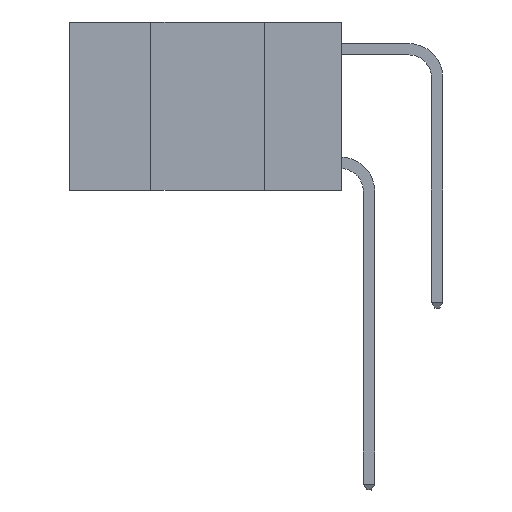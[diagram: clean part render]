
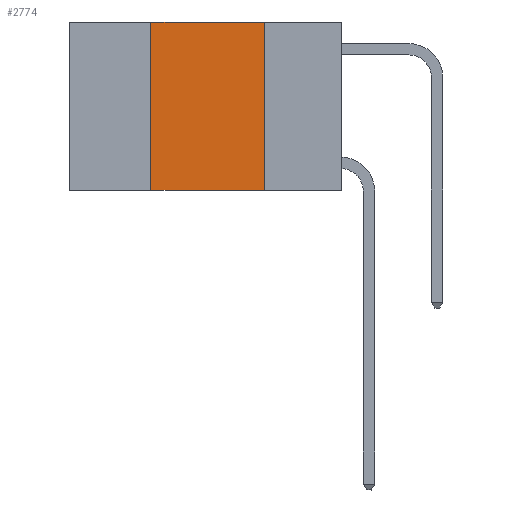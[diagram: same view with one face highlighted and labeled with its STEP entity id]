
A CAD part, left-side view. The second image highlights one B-rep face of the part: STEP entity #2774.
In plain terms, the highlighted planar face has unit normal (-1, 0, 0).
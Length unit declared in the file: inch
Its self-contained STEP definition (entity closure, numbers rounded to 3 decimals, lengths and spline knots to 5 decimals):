
#369 = DIRECTION ( 'NONE',  ( 0., 0., -1. ) ) ;
#434 = CARTESIAN_POINT ( 'NONE',  ( 0., 0.6, 0. ) ) ;
#2393 = LINE ( 'NONE', #25734, #9211 ) ;
#2485 = ORIENTED_EDGE ( 'NONE', *, *, #29262, .F. ) ;
#2774 = ADVANCED_FACE ( 'NONE', ( #15352 ), #8739, .F. ) ;
#2881 = DIRECTION ( 'NONE',  ( 0., 0., 1. ) ) ;
#3376 = CARTESIAN_POINT ( 'NONE',  ( 0., 0.17, 0. ) ) ;
#3693 = DIRECTION ( 'NONE',  ( 1., 0., 0. ) ) ;
#5842 = CARTESIAN_POINT ( 'NONE',  ( 0., 0.6, 0. ) ) ;
#7327 = CARTESIAN_POINT ( 'NONE',  ( 0., 0.42, 0. ) ) ;
#7643 = EDGE_LOOP ( 'NONE', ( #12075, #2485, #14663, #25726 ) ) ;
#8739 = PLANE ( 'NONE',  #21916 ) ;
#9211 = VECTOR ( 'NONE', #28351, 39.37008 ) ;
#10113 = CARTESIAN_POINT ( 'NONE',  ( 0., 0.42, -0.37 ) ) ;
#10222 = EDGE_CURVE ( 'NONE', #17677, #16239, #2393, .T. ) ;
#11270 = VECTOR ( 'NONE', #2881, 39.37008 ) ;
#11651 = VERTEX_POINT ( 'NONE', #15694 ) ;
#12002 = VERTEX_POINT ( 'NONE', #3376 ) ;
#12075 = ORIENTED_EDGE ( 'NONE', *, *, #17034, .F. ) ;
#12296 = EDGE_CURVE ( 'NONE', #17677, #11651, #23474, .T. ) ;
#13211 = VECTOR ( 'NONE', #28980, 39.37008 ) ;
#14426 = VECTOR ( 'NONE', #369, 39.37008 ) ;
#14663 = ORIENTED_EDGE ( 'NONE', *, *, #12296, .F. ) ;
#14830 = LINE ( 'NONE', #434, #13211 ) ;
#15202 = DIRECTION ( 'NONE',  ( 0., 0., -1. ) ) ;
#15352 = FACE_OUTER_BOUND ( 'NONE', #7643, .T. ) ;
#15694 = CARTESIAN_POINT ( 'NONE',  ( 0., 0.42, 0. ) ) ;
#16239 = VERTEX_POINT ( 'NONE', #28101 ) ;
#17034 = EDGE_CURVE ( 'NONE', #12002, #16239, #20672, .T. ) ;
#17677 = VERTEX_POINT ( 'NONE', #10113 ) ;
#20672 = LINE ( 'NONE', #25270, #14426 ) ;
#21916 = AXIS2_PLACEMENT_3D ( 'NONE', #5842, #3693, #15202 ) ;
#23474 = LINE ( 'NONE', #7327, #11270 ) ;
#25270 = CARTESIAN_POINT ( 'NONE',  ( 0., 0.17, 0. ) ) ;
#25726 = ORIENTED_EDGE ( 'NONE', *, *, #10222, .T. ) ;
#25734 = CARTESIAN_POINT ( 'NONE',  ( 0., 0.6, -0.37 ) ) ;
#28101 = CARTESIAN_POINT ( 'NONE',  ( 0., 0.17, -0.37 ) ) ;
#28351 = DIRECTION ( 'NONE',  ( 0., -1., 0. ) ) ;
#28980 = DIRECTION ( 'NONE',  ( 0., -1., 0. ) ) ;
#29262 = EDGE_CURVE ( 'NONE', #11651, #12002, #14830, .T. ) ;
